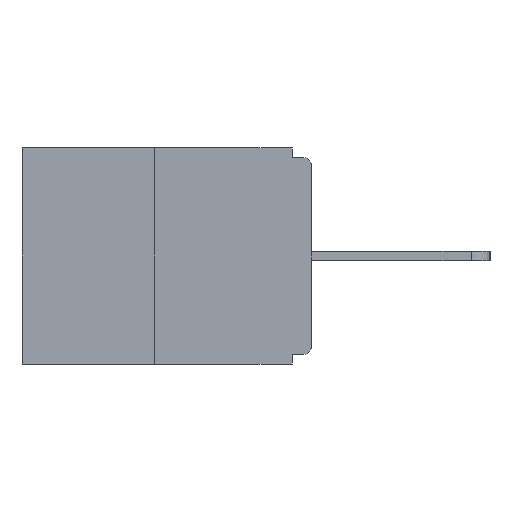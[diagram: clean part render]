
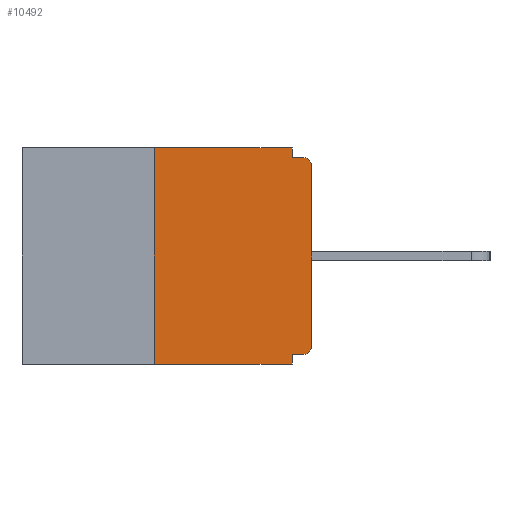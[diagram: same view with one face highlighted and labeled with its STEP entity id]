
A CAD part, left-side view. The second image highlights one B-rep face of the part: STEP entity #10492.
In plain terms, the highlighted planar face has unit normal (-1, 0, 0).
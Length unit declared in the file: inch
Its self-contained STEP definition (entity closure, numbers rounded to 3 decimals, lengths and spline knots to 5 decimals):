
#89 = VERTEX_POINT ( 'NONE', #4826 ) ;
#174 = ORIENTED_EDGE ( 'NONE', *, *, #6571, .F. ) ;
#477 = ORIENTED_EDGE ( 'NONE', *, *, #1129, .T. ) ;
#525 = VECTOR ( 'NONE', #4944, 39.37008 ) ;
#619 = LINE ( 'NONE', #8568, #4489 ) ;
#658 = CARTESIAN_POINT ( 'NONE',  ( 0., 0.031, -0.328 ) ) ;
#1106 = VERTEX_POINT ( 'NONE', #10161 ) ;
#1129 = EDGE_CURVE ( 'NONE', #10180, #5711, #3968, .T. ) ;
#1429 = VECTOR ( 'NONE', #7736, 39.37008 ) ;
#1460 = CARTESIAN_POINT ( 'NONE',  ( 0., 0.031, -0.343 ) ) ;
#1514 = VECTOR ( 'NONE', #1870, 39.37008 ) ;
#1811 = CARTESIAN_POINT ( 'NONE',  ( 0., 0.46, 0. ) ) ;
#1870 = DIRECTION ( 'NONE',  ( 0., 0., 1. ) ) ;
#1997 = LINE ( 'NONE', #6828, #1429 ) ;
#2214 = CIRCLE ( 'NONE', #5758, 0.015 ) ;
#2327 = ORIENTED_EDGE ( 'NONE', *, *, #6016, .F. ) ;
#2338 = EDGE_CURVE ( 'NONE', #1106, #5711, #11199, .T. ) ;
#2638 = CARTESIAN_POINT ( 'NONE',  ( 0., 0.25, -0.343 ) ) ;
#2678 = CARTESIAN_POINT ( 'NONE',  ( 0., 0., -0.03 ) ) ;
#2696 = LINE ( 'NONE', #3809, #5964 ) ;
#2888 = CARTESIAN_POINT ( 'NONE',  ( 0., 0.015, -0.313 ) ) ;
#3573 = CARTESIAN_POINT ( 'NONE',  ( 0., 0.46, 0. ) ) ;
#3606 = DIRECTION ( 'NONE',  ( 0., -1., 0. ) ) ;
#3631 = DIRECTION ( 'NONE',  ( 0., 1., 0. ) ) ;
#3737 = VERTEX_POINT ( 'NONE', #2638 ) ;
#3764 = CARTESIAN_POINT ( 'NONE',  ( 0., 0.015, -0.03 ) ) ;
#3799 = DIRECTION ( 'NONE',  ( -1., 0., 0. ) ) ;
#3809 = CARTESIAN_POINT ( 'NONE',  ( 0., 0.031, 0. ) ) ;
#3901 = DIRECTION ( 'NONE',  ( -1., 0., 0. ) ) ;
#3966 = LINE ( 'NONE', #7937, #1514 ) ;
#3968 = CIRCLE ( 'NONE', #7696, 0.015 ) ;
#4399 = CARTESIAN_POINT ( 'NONE',  ( 0., 0., -0.015 ) ) ;
#4404 = CARTESIAN_POINT ( 'NONE',  ( 0., 0.25, 0. ) ) ;
#4489 = VECTOR ( 'NONE', #3606, 39.37008 ) ;
#4686 = ORIENTED_EDGE ( 'NONE', *, *, #9510, .F. ) ;
#4826 = CARTESIAN_POINT ( 'NONE',  ( 0., 0.015, -0.328 ) ) ;
#4849 = ORIENTED_EDGE ( 'NONE', *, *, #12429, .F. ) ;
#4911 = VECTOR ( 'NONE', #3631, 39.37008 ) ;
#4944 = DIRECTION ( 'NONE',  ( 0., -1., 0. ) ) ;
#4974 = ORIENTED_EDGE ( 'NONE', *, *, #2338, .F. ) ;
#5535 = DIRECTION ( 'NONE',  ( 1., 0., 0. ) ) ;
#5592 = AXIS2_PLACEMENT_3D ( 'NONE', #3573, #5535, #5736 ) ;
#5705 = CARTESIAN_POINT ( 'NONE',  ( 0., 0.031, 0. ) ) ;
#5711 = VERTEX_POINT ( 'NONE', #5827 ) ;
#5736 = DIRECTION ( 'NONE',  ( 0., 0., -1. ) ) ;
#5758 = AXIS2_PLACEMENT_3D ( 'NONE', #2888, #3799, #7772 ) ;
#5827 = CARTESIAN_POINT ( 'NONE',  ( 0., 0.015, -0.015 ) ) ;
#5907 = DIRECTION ( 'NONE',  ( 0., 0., -1. ) ) ;
#5964 = VECTOR ( 'NONE', #5907, 39.37008 ) ;
#6016 = EDGE_CURVE ( 'NONE', #89, #10220, #11111, .T. ) ;
#6127 = EDGE_CURVE ( 'NONE', #8341, #6516, #7744, .T. ) ;
#6401 = VECTOR ( 'NONE', #9261, 39.37008 ) ;
#6466 = FACE_OUTER_BOUND ( 'NONE', #12696, .T. ) ;
#6489 = EDGE_CURVE ( 'NONE', #3737, #8464, #619, .T. ) ;
#6516 = VERTEX_POINT ( 'NONE', #5705 ) ;
#6571 = EDGE_CURVE ( 'NONE', #6516, #1106, #2696, .T. ) ;
#6828 = CARTESIAN_POINT ( 'NONE',  ( 0., 0., 0. ) ) ;
#6948 = EDGE_CURVE ( 'NONE', #89, #12716, #2214, .T. ) ;
#7323 = ORIENTED_EDGE ( 'NONE', *, *, #6127, .F. ) ;
#7525 = LINE ( 'NONE', #1460, #6401 ) ;
#7527 = CARTESIAN_POINT ( 'NONE',  ( 0., 0., -0.313 ) ) ;
#7696 = AXIS2_PLACEMENT_3D ( 'NONE', #3764, #3901, #10625 ) ;
#7736 = DIRECTION ( 'NONE',  ( 0., 0., 1. ) ) ;
#7744 = LINE ( 'NONE', #1811, #525 ) ;
#7772 = DIRECTION ( 'NONE',  ( 0., 0., -1. ) ) ;
#7937 = CARTESIAN_POINT ( 'NONE',  ( 0., 0.25, 0. ) ) ;
#8341 = VERTEX_POINT ( 'NONE', #4404 ) ;
#8363 = DIRECTION ( 'NONE',  ( 0., -1., 0. ) ) ;
#8464 = VERTEX_POINT ( 'NONE', #12445 ) ;
#8568 = CARTESIAN_POINT ( 'NONE',  ( 0., 0.46, -0.343 ) ) ;
#8586 = ORIENTED_EDGE ( 'NONE', *, *, #10975, .T. ) ;
#8760 = VECTOR ( 'NONE', #8363, 39.37008 ) ;
#8992 = ORIENTED_EDGE ( 'NONE', *, *, #6489, .T. ) ;
#9261 = DIRECTION ( 'NONE',  ( 0., 0., -1. ) ) ;
#9510 = EDGE_CURVE ( 'NONE', #10220, #8464, #7525, .T. ) ;
#10161 = CARTESIAN_POINT ( 'NONE',  ( 0., 0.031, -0.015 ) ) ;
#10180 = VERTEX_POINT ( 'NONE', #2678 ) ;
#10220 = VERTEX_POINT ( 'NONE', #658 ) ;
#10310 = CARTESIAN_POINT ( 'NONE',  ( 0., 0., -0.328 ) ) ;
#10447 = PLANE ( 'NONE',  #5592 ) ;
#10492 = ADVANCED_FACE ( 'NONE', ( #6466 ), #10447, .F. ) ;
#10625 = DIRECTION ( 'NONE',  ( 0., 0., -1. ) ) ;
#10975 = EDGE_CURVE ( 'NONE', #12716, #10180, #1997, .T. ) ;
#11111 = LINE ( 'NONE', #10310, #4911 ) ;
#11199 = LINE ( 'NONE', #4399, #8760 ) ;
#12309 = ORIENTED_EDGE ( 'NONE', *, *, #6948, .T. ) ;
#12429 = EDGE_CURVE ( 'NONE', #3737, #8341, #3966, .T. ) ;
#12445 = CARTESIAN_POINT ( 'NONE',  ( 0., 0.031, -0.343 ) ) ;
#12696 = EDGE_LOOP ( 'NONE', ( #7323, #4849, #8992, #4686, #2327, #12309, #8586, #477, #4974, #174 ) ) ;
#12716 = VERTEX_POINT ( 'NONE', #7527 ) ;
